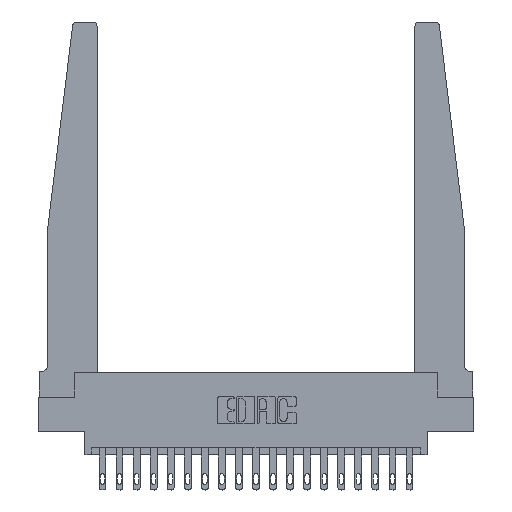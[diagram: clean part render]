
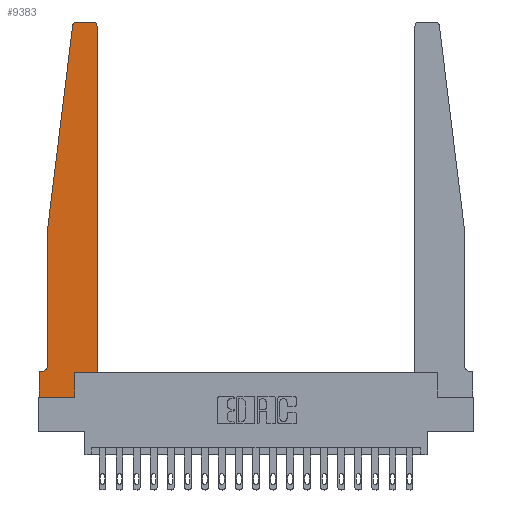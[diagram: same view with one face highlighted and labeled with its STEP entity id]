
A CAD part, top view. The second image highlights one B-rep face of the part: STEP entity #9383.
In plain terms, the highlighted planar face has unit normal (0, 0, 1).
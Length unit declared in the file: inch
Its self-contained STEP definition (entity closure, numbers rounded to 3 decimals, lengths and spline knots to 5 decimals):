
#30 = CARTESIAN_POINT ( 'NONE',  ( 0.27653, 2.72, 0.37 ) ) ;
#159 = VECTOR ( 'NONE', #19115, 39.37008 ) ;
#204 = CARTESIAN_POINT ( 'NONE',  ( 0., 0.1875, 0.37 ) ) ;
#286 = ORIENTED_EDGE ( 'NONE', *, *, #6569, .T. ) ;
#306 = VECTOR ( 'NONE', #7441, 39.37008 ) ;
#308 = PLANE ( 'NONE',  #5212 ) ;
#992 = CARTESIAN_POINT ( 'NONE',  ( 0.425, 0.18, 0.37 ) ) ;
#1758 = VECTOR ( 'NONE', #5580, 39.37008 ) ;
#1924 = CARTESIAN_POINT ( 'NONE',  ( 0.065, 1.25, 0.37 ) ) ;
#1929 = DIRECTION ( 'NONE',  ( 0., 1., 0. ) ) ;
#2162 = EDGE_CURVE ( 'NONE', #9771, #7112, #5884, .T. ) ;
#2514 = EDGE_CURVE ( 'NONE', #12419, #14197, #12448, .T. ) ;
#2612 = VECTOR ( 'NONE', #9318, 39.37008 ) ;
#3044 = CARTESIAN_POINT ( 'NONE',  ( 0.015, 0.2375, 0.37 ) ) ;
#3097 = ORIENTED_EDGE ( 'NONE', *, *, #3797, .T. ) ;
#3175 = DIRECTION ( 'NONE',  ( 0., 0., 1. ) ) ;
#3529 = VECTOR ( 'NONE', #20550, 39.37008 ) ;
#3585 = VECTOR ( 'NONE', #20620, 39.37008 ) ;
#3797 = EDGE_CURVE ( 'NONE', #7112, #19735, #12348, .T. ) ;
#3988 = VERTEX_POINT ( 'NONE', #10425 ) ;
#4180 = EDGE_CURVE ( 'NONE', #4590, #12419, #20316, .T. ) ;
#4541 = VECTOR ( 'NONE', #17425, 39.37008 ) ;
#4590 = VERTEX_POINT ( 'NONE', #5704 ) ;
#4638 = DIRECTION ( 'NONE',  ( -1., 0., 0. ) ) ;
#4718 = CARTESIAN_POINT ( 'NONE',  ( 0.425, 0.18, 0.37 ) ) ;
#5042 = CARTESIAN_POINT ( 'NONE',  ( 0., 0., 0.37 ) ) ;
#5212 = AXIS2_PLACEMENT_3D ( 'NONE', #204, #16299, #18081 ) ;
#5266 = CARTESIAN_POINT ( 'NONE',  ( 0.24675, 2.72367, 0.37 ) ) ;
#5580 = DIRECTION ( 'NONE',  ( -0.122, -0.992, 0. ) ) ;
#5609 = EDGE_CURVE ( 'NONE', #11516, #13675, #10773, .T. ) ;
#5704 = CARTESIAN_POINT ( 'NONE',  ( 0.015, 0.1875, 0.37 ) ) ;
#5884 = LINE ( 'NONE', #14152, #306 ) ;
#5948 = ORIENTED_EDGE ( 'NONE', *, *, #6140, .T. ) ;
#6140 = EDGE_CURVE ( 'NONE', #11053, #8588, #7252, .T. ) ;
#6530 = EDGE_CURVE ( 'NONE', #8588, #12785, #11428, .T. ) ;
#6569 = EDGE_CURVE ( 'NONE', #14197, #9771, #19415, .T. ) ;
#7112 = VERTEX_POINT ( 'NONE', #11719 ) ;
#7252 = LINE ( 'NONE', #8587, #1758 ) ;
#7318 = CIRCLE ( 'NONE', #15036, 0.03 ) ;
#7326 = CARTESIAN_POINT ( 'NONE',  ( 0.065, 0.2375, 0.37 ) ) ;
#7441 = DIRECTION ( 'NONE',  ( 0., 1., 0. ) ) ;
#7700 = AXIS2_PLACEMENT_3D ( 'NONE', #3044, #8278, #4638 ) ;
#7723 = EDGE_CURVE ( 'NONE', #13675, #3988, #13737, .T. ) ;
#8154 = CARTESIAN_POINT ( 'NONE',  ( 0.2605, 0., 0.37 ) ) ;
#8278 = DIRECTION ( 'NONE',  ( 0., 0., -1. ) ) ;
#8300 = VECTOR ( 'NONE', #1929, 39.37008 ) ;
#8587 = CARTESIAN_POINT ( 'NONE',  ( 0.065, 1.25, 0.37 ) ) ;
#8588 = VERTEX_POINT ( 'NONE', #1924 ) ;
#8713 = ORIENTED_EDGE ( 'NONE', *, *, #4180, .T. ) ;
#8833 = ORIENTED_EDGE ( 'NONE', *, *, #7723, .T. ) ;
#8977 = CARTESIAN_POINT ( 'NONE',  ( 0., 0., 0.37 ) ) ;
#9318 = DIRECTION ( 'NONE',  ( -1., 0., 0. ) ) ;
#9383 = ADVANCED_FACE ( 'NONE', ( #19349 ), #308, .T. ) ;
#9661 = CARTESIAN_POINT ( 'NONE',  ( 0.395, 2.75, 0.37 ) ) ;
#9771 = VERTEX_POINT ( 'NONE', #8154 ) ;
#10017 = CIRCLE ( 'NONE', #7700, 0.05 ) ;
#10425 = CARTESIAN_POINT ( 'NONE',  ( 0.27653, 2.75, 0.37 ) ) ;
#10773 = CIRCLE ( 'NONE', #16495, 0.03 ) ;
#11053 = VERTEX_POINT ( 'NONE', #5266 ) ;
#11367 = DIRECTION ( 'NONE',  ( 1., 0., 0. ) ) ;
#11428 = LINE ( 'NONE', #12591, #4541 ) ;
#11516 = VERTEX_POINT ( 'NONE', #16777 ) ;
#11719 = CARTESIAN_POINT ( 'NONE',  ( 0.2605, 0.18, 0.37 ) ) ;
#11794 = ORIENTED_EDGE ( 'NONE', *, *, #6530, .T. ) ;
#12348 = LINE ( 'NONE', #992, #3529 ) ;
#12419 = VERTEX_POINT ( 'NONE', #14193 ) ;
#12448 = LINE ( 'NONE', #8977, #14151 ) ;
#12480 = ORIENTED_EDGE ( 'NONE', *, *, #2162, .T. ) ;
#12591 = CARTESIAN_POINT ( 'NONE',  ( 0.065, 1.25, 0.37 ) ) ;
#12785 = VERTEX_POINT ( 'NONE', #7326 ) ;
#13675 = VERTEX_POINT ( 'NONE', #9661 ) ;
#13737 = LINE ( 'NONE', #15444, #2612 ) ;
#14151 = VECTOR ( 'NONE', #15808, 39.37008 ) ;
#14152 = CARTESIAN_POINT ( 'NONE',  ( 0.2605, 0.18, 0.37 ) ) ;
#14193 = CARTESIAN_POINT ( 'NONE',  ( 0., 0.1875, 0.37 ) ) ;
#14197 = VERTEX_POINT ( 'NONE', #18015 ) ;
#14221 = DIRECTION ( 'NONE',  ( 0., 0., 1. ) ) ;
#14747 = EDGE_CURVE ( 'NONE', #3988, #11053, #7318, .T. ) ;
#15036 = AXIS2_PLACEMENT_3D ( 'NONE', #30, #14221, #19176 ) ;
#15444 = CARTESIAN_POINT ( 'NONE',  ( 0.25, 2.75, 0.37 ) ) ;
#15784 = CARTESIAN_POINT ( 'NONE',  ( 0.065, 0.1875, 0.37 ) ) ;
#15808 = DIRECTION ( 'NONE',  ( 0., -1., 0. ) ) ;
#16210 = CARTESIAN_POINT ( 'NONE',  ( 0.395, 2.72, 0.37 ) ) ;
#16299 = DIRECTION ( 'NONE',  ( 0., 0., 1. ) ) ;
#16356 = CARTESIAN_POINT ( 'NONE',  ( 0.425, 0.18, 0.37 ) ) ;
#16424 = ORIENTED_EDGE ( 'NONE', *, *, #19445, .T. ) ;
#16495 = AXIS2_PLACEMENT_3D ( 'NONE', #16210, #3175, #11367 ) ;
#16661 = ORIENTED_EDGE ( 'NONE', *, *, #17529, .T. ) ;
#16777 = CARTESIAN_POINT ( 'NONE',  ( 0.425, 2.72, 0.37 ) ) ;
#17425 = DIRECTION ( 'NONE',  ( 0., -1., 0. ) ) ;
#17529 = EDGE_CURVE ( 'NONE', #19735, #11516, #17939, .T. ) ;
#17939 = LINE ( 'NONE', #16356, #8300 ) ;
#18015 = CARTESIAN_POINT ( 'NONE',  ( 0., 0., 0.37 ) ) ;
#18081 = DIRECTION ( 'NONE',  ( 1., 0., 0. ) ) ;
#19115 = DIRECTION ( 'NONE',  ( 1., 0., 0. ) ) ;
#19176 = DIRECTION ( 'NONE',  ( 1., 0., 0. ) ) ;
#19349 = FACE_OUTER_BOUND ( 'NONE', #20587, .T. ) ;
#19415 = LINE ( 'NONE', #5042, #159 ) ;
#19445 = EDGE_CURVE ( 'NONE', #12785, #4590, #10017, .T. ) ;
#19735 = VERTEX_POINT ( 'NONE', #4718 ) ;
#19746 = ORIENTED_EDGE ( 'NONE', *, *, #5609, .T. ) ;
#19837 = ORIENTED_EDGE ( 'NONE', *, *, #2514, .T. ) ;
#20316 = LINE ( 'NONE', #15784, #3585 ) ;
#20549 = ORIENTED_EDGE ( 'NONE', *, *, #14747, .T. ) ;
#20550 = DIRECTION ( 'NONE',  ( 1., 0., 0. ) ) ;
#20587 = EDGE_LOOP ( 'NONE', ( #8833, #20549, #5948, #11794, #16424, #8713, #19837, #286, #12480, #3097, #16661, #19746 ) ) ;
#20620 = DIRECTION ( 'NONE',  ( -1., 0., 0. ) ) ;
